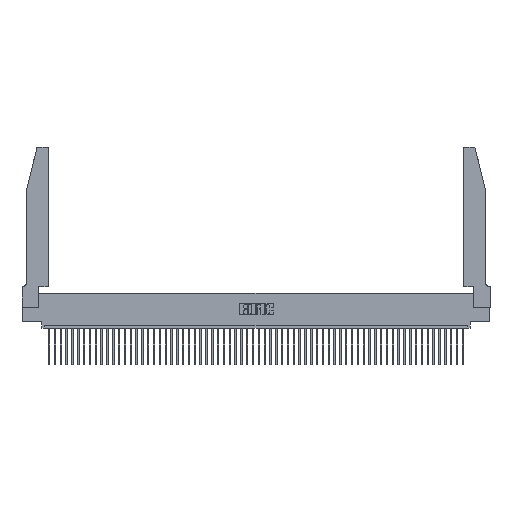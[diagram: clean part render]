
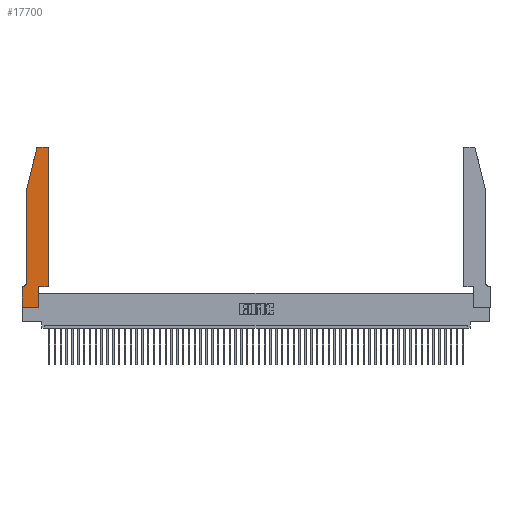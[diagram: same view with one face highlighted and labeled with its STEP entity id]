
A CAD part, top view. The second image highlights one B-rep face of the part: STEP entity #17700.
In plain terms, the highlighted planar face has unit normal (0, 0, 1).
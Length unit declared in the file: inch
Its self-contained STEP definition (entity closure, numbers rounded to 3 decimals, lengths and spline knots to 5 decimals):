
#198 = ORIENTED_EDGE ( 'NONE', *, *, #22099, .T. ) ;
#412 = VERTEX_POINT ( 'NONE', #29922 ) ;
#917 = CARTESIAN_POINT ( 'NONE',  ( 0.0755, 0.35, 0.37 ) ) ;
#1104 = EDGE_CURVE ( 'NONE', #7052, #45556, #24805, .T. ) ;
#2210 = EDGE_CURVE ( 'NONE', #3351, #7052, #6059, .T. ) ;
#2261 = ORIENTED_EDGE ( 'NONE', *, *, #45726, .T. ) ;
#2494 = EDGE_CURVE ( 'NONE', #31052, #20133, #4078, .T. ) ;
#2934 = CARTESIAN_POINT ( 'NONE',  ( 0.4505, 0.35, 0.37 ) ) ;
#3351 = VERTEX_POINT ( 'NONE', #44345 ) ;
#3442 = VECTOR ( 'NONE', #13761, 39.37008 ) ;
#4078 = CIRCLE ( 'NONE', #41094, 0.03 ) ;
#4251 = CARTESIAN_POINT ( 'NONE',  ( 0.284, 2.75, 0.37 ) ) ;
#5454 = EDGE_CURVE ( 'NONE', #39133, #412, #30176, .T. ) ;
#5843 = ORIENTED_EDGE ( 'NONE', *, *, #24050, .T. ) ;
#5872 = LINE ( 'NONE', #47908, #17756 ) ;
#6006 = VECTOR ( 'NONE', #37390, 39.37008 ) ;
#6059 = LINE ( 'NONE', #917, #3442 ) ;
#7052 = VERTEX_POINT ( 'NONE', #23864 ) ;
#7127 = CARTESIAN_POINT ( 'NONE',  ( 0.2605, 2.75, 0.37 ) ) ;
#8583 = VECTOR ( 'NONE', #14956, 39.37008 ) ;
#8840 = LINE ( 'NONE', #54672, #45483 ) ;
#10039 = ORIENTED_EDGE ( 'NONE', *, *, #48299, .T. ) ;
#10675 = CARTESIAN_POINT ( 'NONE',  ( 0.2865, 0.35, 0.37 ) ) ;
#11671 = PLANE ( 'NONE',  #48828 ) ;
#12205 = EDGE_CURVE ( 'NONE', #20133, #50562, #45323, .T. ) ;
#13589 = VERTEX_POINT ( 'NONE', #41373 ) ;
#13761 = DIRECTION ( 'NONE',  ( -1., 0., 0. ) ) ;
#13805 = ORIENTED_EDGE ( 'NONE', *, *, #1104, .T. ) ;
#14956 = DIRECTION ( 'NONE',  ( 0., 1., 0. ) ) ;
#15258 = LINE ( 'NONE', #10675, #8583 ) ;
#16564 = EDGE_CURVE ( 'NONE', #25239, #3351, #30108, .T. ) ;
#17362 = ORIENTED_EDGE ( 'NONE', *, *, #48052, .T. ) ;
#17700 = ADVANCED_FACE ( 'NONE', ( #36754 ), #11671, .T. ) ;
#17756 = VECTOR ( 'NONE', #50400, 39.37008 ) ;
#18261 = CARTESIAN_POINT ( 'NONE',  ( 0.0755, 2., 0.37 ) ) ;
#18503 = DIRECTION ( 'NONE',  ( 0., 0., 1. ) ) ;
#18926 = VECTOR ( 'NONE', #37667, 39.37008 ) ;
#20128 = DIRECTION ( 'NONE',  ( 0., 0., 1. ) ) ;
#20133 = VERTEX_POINT ( 'NONE', #30692 ) ;
#20536 = CARTESIAN_POINT ( 'NONE',  ( 0.0055, 0.42, 0.37 ) ) ;
#21457 = ORIENTED_EDGE ( 'NONE', *, *, #2494, .T. ) ;
#21811 = CARTESIAN_POINT ( 'NONE',  ( 0.0755, 2., 0.37 ) ) ;
#21914 = DIRECTION ( 'NONE',  ( 1., 0., 0. ) ) ;
#21939 = ORIENTED_EDGE ( 'NONE', *, *, #5454, .T. ) ;
#22099 = EDGE_CURVE ( 'NONE', #46452, #31052, #53204, .T. ) ;
#23864 = CARTESIAN_POINT ( 'NONE',  ( 0., 0.35, 0.37 ) ) ;
#24050 = EDGE_CURVE ( 'NONE', #47706, #39133, #5872, .T. ) ;
#24449 = DIRECTION ( 'NONE',  ( -1., 0., 0. ) ) ;
#24805 = LINE ( 'NONE', #32403, #34073 ) ;
#25239 = VERTEX_POINT ( 'NONE', #27196 ) ;
#27196 = CARTESIAN_POINT ( 'NONE',  ( 0.0755, 0.42, 0.37 ) ) ;
#27899 = CARTESIAN_POINT ( 'NONE',  ( 0.284, 2.72, 0.37 ) ) ;
#28302 = DIRECTION ( 'NONE',  ( 0., 0., -1. ) ) ;
#28732 = EDGE_CURVE ( 'NONE', #50562, #25239, #48791, .T. ) ;
#29901 = AXIS2_PLACEMENT_3D ( 'NONE', #35767, #18503, #52857 ) ;
#29922 = CARTESIAN_POINT ( 'NONE',  ( 0.4505, 2.72, 0.37 ) ) ;
#30108 = CIRCLE ( 'NONE', #44541, 0.07 ) ;
#30176 = LINE ( 'NONE', #2934, #18926 ) ;
#30315 = DIRECTION ( 'NONE',  ( 0., -1., 0. ) ) ;
#30692 = CARTESIAN_POINT ( 'NONE',  ( 0.25487, 2.72718, 0.37 ) ) ;
#31052 = VERTEX_POINT ( 'NONE', #4251 ) ;
#31087 = CARTESIAN_POINT ( 'NONE',  ( 0.0755, 2., 0.37 ) ) ;
#31985 = VECTOR ( 'NONE', #39855, 39.37008 ) ;
#32403 = CARTESIAN_POINT ( 'NONE',  ( 0., 0., 0.37 ) ) ;
#32676 = EDGE_LOOP ( 'NONE', ( #198, #21457, #35708, #51272, #43419, #44719, #13805, #17362, #2261, #5843, #21939, #10039 ) ) ;
#34073 = VECTOR ( 'NONE', #54003, 39.37008 ) ;
#34451 = CARTESIAN_POINT ( 'NONE',  ( 0.4205, 2.75, 0.37 ) ) ;
#35708 = ORIENTED_EDGE ( 'NONE', *, *, #12205, .T. ) ;
#35767 = CARTESIAN_POINT ( 'NONE',  ( 0.4205, 2.72, 0.37 ) ) ;
#36560 = CARTESIAN_POINT ( 'NONE',  ( 0., 0.35, 0.37 ) ) ;
#36754 = FACE_OUTER_BOUND ( 'NONE', #32676, .T. ) ;
#37390 = DIRECTION ( 'NONE',  ( -1., 0., 0. ) ) ;
#37667 = DIRECTION ( 'NONE',  ( 0., 1., 0. ) ) ;
#38069 = CARTESIAN_POINT ( 'NONE',  ( 0., 0., 0.37 ) ) ;
#39133 = VERTEX_POINT ( 'NONE', #46204 ) ;
#39855 = DIRECTION ( 'NONE',  ( -0.239, -0.971, 0. ) ) ;
#39922 = CARTESIAN_POINT ( 'NONE',  ( 0.2865, 0.35, 0.37 ) ) ;
#41094 = AXIS2_PLACEMENT_3D ( 'NONE', #27899, #20128, #49677 ) ;
#41373 = CARTESIAN_POINT ( 'NONE',  ( 0.2865, 0., 0.37 ) ) ;
#43419 = ORIENTED_EDGE ( 'NONE', *, *, #16564, .T. ) ;
#44345 = CARTESIAN_POINT ( 'NONE',  ( 0.0055, 0.35, 0.37 ) ) ;
#44541 = AXIS2_PLACEMENT_3D ( 'NONE', #20536, #28302, #24449 ) ;
#44719 = ORIENTED_EDGE ( 'NONE', *, *, #2210, .T. ) ;
#45323 = LINE ( 'NONE', #31087, #31985 ) ;
#45483 = VECTOR ( 'NONE', #55042, 39.37008 ) ;
#45553 = VECTOR ( 'NONE', #30315, 39.37008 ) ;
#45556 = VERTEX_POINT ( 'NONE', #38069 ) ;
#45726 = EDGE_CURVE ( 'NONE', #13589, #47706, #15258, .T. ) ;
#46185 = CIRCLE ( 'NONE', #29901, 0.03 ) ;
#46204 = CARTESIAN_POINT ( 'NONE',  ( 0.4505, 0.35, 0.37 ) ) ;
#46452 = VERTEX_POINT ( 'NONE', #34451 ) ;
#47706 = VERTEX_POINT ( 'NONE', #39922 ) ;
#47908 = CARTESIAN_POINT ( 'NONE',  ( 0.4505, 0.35, 0.37 ) ) ;
#48052 = EDGE_CURVE ( 'NONE', #45556, #13589, #8840, .T. ) ;
#48299 = EDGE_CURVE ( 'NONE', #412, #46452, #46185, .T. ) ;
#48791 = LINE ( 'NONE', #21811, #45553 ) ;
#48828 = AXIS2_PLACEMENT_3D ( 'NONE', #36560, #51454, #21914 ) ;
#49677 = DIRECTION ( 'NONE',  ( 1., 0., 0. ) ) ;
#50400 = DIRECTION ( 'NONE',  ( 1., 0., 0. ) ) ;
#50562 = VERTEX_POINT ( 'NONE', #18261 ) ;
#51272 = ORIENTED_EDGE ( 'NONE', *, *, #28732, .T. ) ;
#51454 = DIRECTION ( 'NONE',  ( 0., 0., 1. ) ) ;
#52857 = DIRECTION ( 'NONE',  ( 1., 0., 0. ) ) ;
#53204 = LINE ( 'NONE', #7127, #6006 ) ;
#54003 = DIRECTION ( 'NONE',  ( 0., -1., 0. ) ) ;
#54672 = CARTESIAN_POINT ( 'NONE',  ( 0., 0., 0.37 ) ) ;
#55042 = DIRECTION ( 'NONE',  ( 1., 0., 0. ) ) ;
